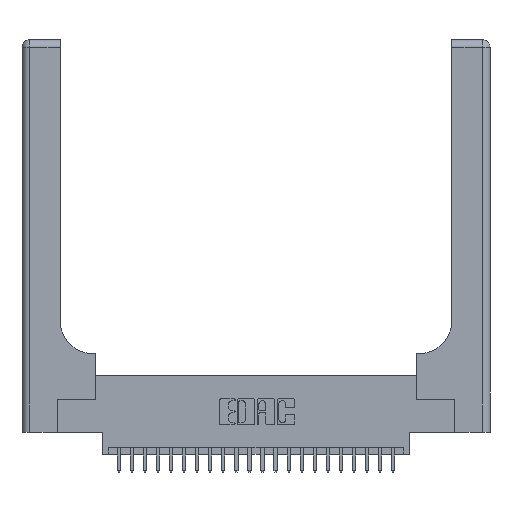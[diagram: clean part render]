
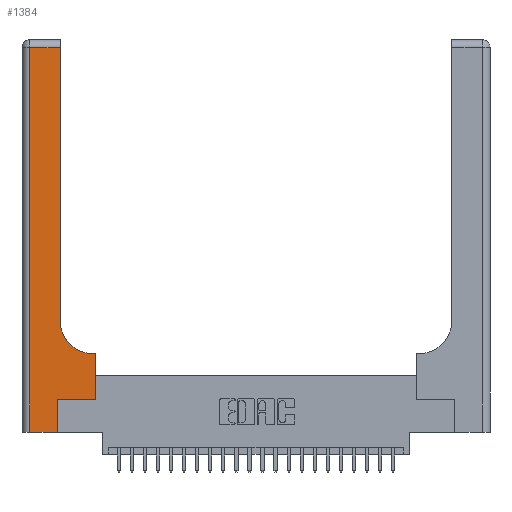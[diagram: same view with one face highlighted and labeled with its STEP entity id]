
A CAD part, top view. The second image highlights one B-rep face of the part: STEP entity #1384.
In plain terms, the highlighted planar face has unit normal (0, 0, 1).
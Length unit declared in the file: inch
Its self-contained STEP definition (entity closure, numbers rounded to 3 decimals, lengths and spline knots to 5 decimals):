
#534 = EDGE_CURVE ( 'NONE', #17543, #21150, #19686, .T. ) ;
#662 = VERTEX_POINT ( 'NONE', #12565 ) ;
#1384 = ADVANCED_FACE ( 'NONE', ( #24254 ), #19176, .F. ) ;
#1569 = CARTESIAN_POINT ( 'NONE',  ( 0.5415, 0.6, 0.37 ) ) ;
#1644 = DIRECTION ( 'NONE',  ( 0., 1., 0. ) ) ;
#2007 = LINE ( 'NONE', #13959, #17243 ) ;
#2063 = DIRECTION ( 'NONE',  ( -1., 0., 0. ) ) ;
#2310 = DIRECTION ( 'NONE',  ( -1., 0., 0. ) ) ;
#2571 = VERTEX_POINT ( 'NONE', #7005 ) ;
#2600 = CARTESIAN_POINT ( 'NONE',  ( 0.06, 3., 0.37 ) ) ;
#2708 = ORIENTED_EDGE ( 'NONE', *, *, #18456, .T. ) ;
#2907 = CARTESIAN_POINT ( 'NONE',  ( 0.5585, 0.6, 0.37 ) ) ;
#3280 = ORIENTED_EDGE ( 'NONE', *, *, #8386, .T. ) ;
#3533 = VECTOR ( 'NONE', #4816, 39.37008 ) ;
#3972 = AXIS2_PLACEMENT_3D ( 'NONE', #23116, #20626, #13103 ) ;
#4145 = LINE ( 'NONE', #2600, #3533 ) ;
#4366 = LINE ( 'NONE', #20095, #5572 ) ;
#4492 = CARTESIAN_POINT ( 'NONE',  ( 0.2915, 2.94, 0.37 ) ) ;
#4758 = VECTOR ( 'NONE', #12457, 39.37008 ) ;
#4812 = EDGE_CURVE ( 'NONE', #21150, #8195, #23054, .T. ) ;
#4816 = DIRECTION ( 'NONE',  ( 0., -1., 0. ) ) ;
#5330 = CARTESIAN_POINT ( 'NONE',  ( 0.2915, 3., 0.37 ) ) ;
#5572 = VECTOR ( 'NONE', #12216, 39.37008 ) ;
#5833 = CARTESIAN_POINT ( 'NONE',  ( 0.5415, 0.85, 0.37 ) ) ;
#6875 = LINE ( 'NONE', #13048, #20600 ) ;
#6993 = VERTEX_POINT ( 'NONE', #17536 ) ;
#7005 = CARTESIAN_POINT ( 'NONE',  ( 0.06, 0., 0.37 ) ) ;
#7321 = ORIENTED_EDGE ( 'NONE', *, *, #4812, .T. ) ;
#7678 = VERTEX_POINT ( 'NONE', #10774 ) ;
#7801 = DIRECTION ( 'NONE',  ( 0., 1., 0. ) ) ;
#8080 = LINE ( 'NONE', #23732, #19086 ) ;
#8099 = ORIENTED_EDGE ( 'NONE', *, *, #534, .T. ) ;
#8195 = VERTEX_POINT ( 'NONE', #4492 ) ;
#8282 = EDGE_CURVE ( 'NONE', #7678, #6993, #9901, .T. ) ;
#8285 = CARTESIAN_POINT ( 'NONE',  ( 0.269, 0.25, 0.37 ) ) ;
#8311 = EDGE_CURVE ( 'NONE', #12716, #2571, #4145, .T. ) ;
#8375 = VECTOR ( 'NONE', #7801, 39.37008 ) ;
#8386 = EDGE_CURVE ( 'NONE', #6993, #8539, #6875, .T. ) ;
#8539 = VERTEX_POINT ( 'NONE', #2907 ) ;
#9687 = ORIENTED_EDGE ( 'NONE', *, *, #8311, .T. ) ;
#9829 = EDGE_CURVE ( 'NONE', #2571, #662, #4366, .T. ) ;
#9847 = EDGE_LOOP ( 'NONE', ( #7321, #19935, #9687, #17820, #2708, #23705, #3280, #10987, #8099 ) ) ;
#9901 = LINE ( 'NONE', #8285, #4758 ) ;
#10774 = CARTESIAN_POINT ( 'NONE',  ( 0.269, 0.25, 0.37 ) ) ;
#10987 = ORIENTED_EDGE ( 'NONE', *, *, #15174, .T. ) ;
#11567 = CARTESIAN_POINT ( 'NONE',  ( 0.06, 2.94, 0.37 ) ) ;
#12216 = DIRECTION ( 'NONE',  ( 1., 0., 0. ) ) ;
#12457 = DIRECTION ( 'NONE',  ( 1., 0., 0. ) ) ;
#12565 = CARTESIAN_POINT ( 'NONE',  ( 0.269, 0., 0.37 ) ) ;
#12716 = VERTEX_POINT ( 'NONE', #11567 ) ;
#13048 = CARTESIAN_POINT ( 'NONE',  ( 0.5585, 0.25, 0.37 ) ) ;
#13103 = DIRECTION ( 'NONE',  ( -1., 0., 0. ) ) ;
#13347 = DIRECTION ( 'NONE',  ( 0., 0., -1. ) ) ;
#13754 = CARTESIAN_POINT ( 'NONE',  ( 0.269, 0., 0.37 ) ) ;
#13959 = CARTESIAN_POINT ( 'NONE',  ( 0., 2.94, 0.37 ) ) ;
#14889 = DIRECTION ( 'NONE',  ( 0., 1., 0. ) ) ;
#15174 = EDGE_CURVE ( 'NONE', #8539, #17543, #8080, .T. ) ;
#16932 = VECTOR ( 'NONE', #14889, 39.37008 ) ;
#17243 = VECTOR ( 'NONE', #2310, 39.37008 ) ;
#17276 = DIRECTION ( 'NONE',  ( 1., 0., 0. ) ) ;
#17536 = CARTESIAN_POINT ( 'NONE',  ( 0.5585, 0.25, 0.37 ) ) ;
#17543 = VERTEX_POINT ( 'NONE', #1569 ) ;
#17820 = ORIENTED_EDGE ( 'NONE', *, *, #9829, .T. ) ;
#18002 = AXIS2_PLACEMENT_3D ( 'NONE', #5833, #13347, #17276 ) ;
#18139 = CARTESIAN_POINT ( 'NONE',  ( 0.2915, 0.85, 0.37 ) ) ;
#18456 = EDGE_CURVE ( 'NONE', #662, #7678, #21214, .T. ) ;
#19086 = VECTOR ( 'NONE', #2063, 39.37008 ) ;
#19176 = PLANE ( 'NONE',  #3972 ) ;
#19686 = CIRCLE ( 'NONE', #18002, 0.25 ) ;
#19935 = ORIENTED_EDGE ( 'NONE', *, *, #25058, .T. ) ;
#20095 = CARTESIAN_POINT ( 'NONE',  ( 0., 0., 0.37 ) ) ;
#20600 = VECTOR ( 'NONE', #1644, 39.37008 ) ;
#20626 = DIRECTION ( 'NONE',  ( 0., 0., -1. ) ) ;
#21150 = VERTEX_POINT ( 'NONE', #18139 ) ;
#21214 = LINE ( 'NONE', #13754, #8375 ) ;
#23054 = LINE ( 'NONE', #5330, #16932 ) ;
#23116 = CARTESIAN_POINT ( 'NONE',  ( 0., 3., 0.37 ) ) ;
#23705 = ORIENTED_EDGE ( 'NONE', *, *, #8282, .T. ) ;
#23732 = CARTESIAN_POINT ( 'NONE',  ( 0.2915, 0.6, 0.37 ) ) ;
#24254 = FACE_OUTER_BOUND ( 'NONE', #9847, .T. ) ;
#25058 = EDGE_CURVE ( 'NONE', #8195, #12716, #2007, .T. ) ;
